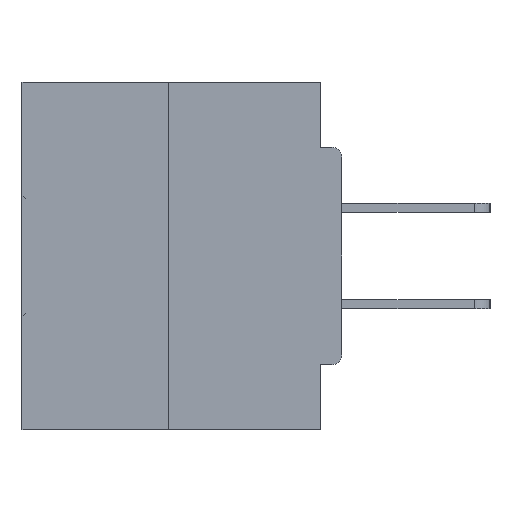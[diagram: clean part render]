
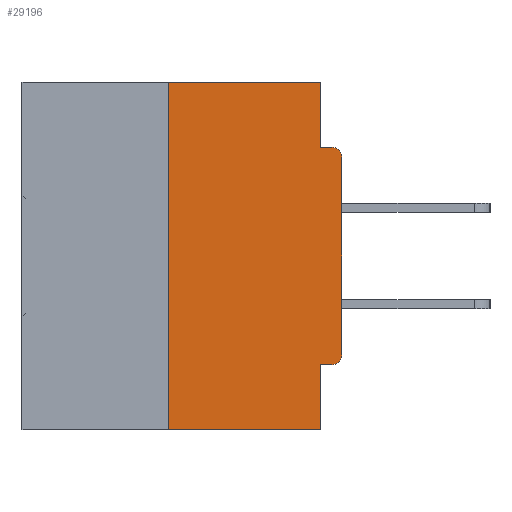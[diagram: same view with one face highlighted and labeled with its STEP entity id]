
A CAD part, left-side view. The second image highlights one B-rep face of the part: STEP entity #29196.
In plain terms, the highlighted planar face has unit normal (-1, 0, 0).
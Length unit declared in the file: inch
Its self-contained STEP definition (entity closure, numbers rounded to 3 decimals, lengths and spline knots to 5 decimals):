
#55 = FACE_OUTER_BOUND ( 'NONE', #29876, .T. ) ;
#307 = VERTEX_POINT ( 'NONE', #12063 ) ;
#422 = VECTOR ( 'NONE', #13585, 39.37008 ) ;
#496 = DIRECTION ( 'NONE',  ( 0., 0., -1. ) ) ;
#652 = CARTESIAN_POINT ( 'NONE',  ( 0., 0.031, 0. ) ) ;
#930 = LINE ( 'NONE', #10908, #422 ) ;
#2035 = DIRECTION ( 'NONE',  ( -1., 0., 0. ) ) ;
#3296 = ORIENTED_EDGE ( 'NONE', *, *, #38791, .F. ) ;
#4219 = EDGE_CURVE ( 'NONE', #8101, #42566, #31066, .T. ) ;
#5062 = ORIENTED_EDGE ( 'NONE', *, *, #29926, .T. ) ;
#5586 = DIRECTION ( 'NONE',  ( 0., 0., -1. ) ) ;
#6471 = DIRECTION ( 'NONE',  ( 1., 0., 0. ) ) ;
#7064 = LINE ( 'NONE', #11049, #9566 ) ;
#7472 = VECTOR ( 'NONE', #21072, 39.37008 ) ;
#7932 = ORIENTED_EDGE ( 'NONE', *, *, #4219, .F. ) ;
#7961 = VERTEX_POINT ( 'NONE', #36113 ) ;
#7991 = DIRECTION ( 'NONE',  ( 0., 1., 0. ) ) ;
#8101 = VERTEX_POINT ( 'NONE', #23896 ) ;
#8283 = CARTESIAN_POINT ( 'NONE',  ( 0., 0.015, -0.0935 ) ) ;
#8564 = VERTEX_POINT ( 'NONE', #42019 ) ;
#8999 = CARTESIAN_POINT ( 'NONE',  ( 0., 0., 0. ) ) ;
#9387 = CIRCLE ( 'NONE', #21454, 0.015 ) ;
#9566 = VECTOR ( 'NONE', #41046, 39.37008 ) ;
#9728 = CARTESIAN_POINT ( 'NONE',  ( 0., 0.031, -0.5 ) ) ;
#9814 = DIRECTION ( 'NONE',  ( -1., 0., 0. ) ) ;
#9816 = VERTEX_POINT ( 'NONE', #8283 ) ;
#10243 = LINE ( 'NONE', #39801, #36415 ) ;
#10625 = VERTEX_POINT ( 'NONE', #31506 ) ;
#10864 = VECTOR ( 'NONE', #35394, 39.37008 ) ;
#10908 = CARTESIAN_POINT ( 'NONE',  ( 0., 0., -0.0935 ) ) ;
#11049 = CARTESIAN_POINT ( 'NONE',  ( 0., 0.25, 0. ) ) ;
#12063 = CARTESIAN_POINT ( 'NONE',  ( 0., 0., -0.3915 ) ) ;
#12364 = ORIENTED_EDGE ( 'NONE', *, *, #25014, .F. ) ;
#13346 = CARTESIAN_POINT ( 'NONE',  ( 0., 0.031, -0.5 ) ) ;
#13406 = EDGE_CURVE ( 'NONE', #42566, #9816, #930, .T. ) ;
#13421 = LINE ( 'NONE', #20533, #18988 ) ;
#13585 = DIRECTION ( 'NONE',  ( 0., -1., 0. ) ) ;
#13755 = ORIENTED_EDGE ( 'NONE', *, *, #36612, .F. ) ;
#16016 = ORIENTED_EDGE ( 'NONE', *, *, #32599, .F. ) ;
#16123 = DIRECTION ( 'NONE',  ( 0., 0., 1. ) ) ;
#16405 = LINE ( 'NONE', #9728, #33679 ) ;
#16942 = PLANE ( 'NONE',  #22169 ) ;
#17149 = DIRECTION ( 'NONE',  ( 0., 0., -1. ) ) ;
#18069 = CARTESIAN_POINT ( 'NONE',  ( 0., 0.25, -0.5 ) ) ;
#18296 = AXIS2_PLACEMENT_3D ( 'NONE', #42648, #2035, #5586 ) ;
#18988 = VECTOR ( 'NONE', #7991, 39.37008 ) ;
#19412 = LINE ( 'NONE', #21879, #10864 ) ;
#20533 = CARTESIAN_POINT ( 'NONE',  ( 0., 0., -0.4065 ) ) ;
#20897 = VERTEX_POINT ( 'NONE', #13346 ) ;
#21072 = DIRECTION ( 'NONE',  ( 0., 0., -1. ) ) ;
#21454 = AXIS2_PLACEMENT_3D ( 'NONE', #26690, #9814, #17149 ) ;
#21879 = CARTESIAN_POINT ( 'NONE',  ( 0., 0.46, -0.5 ) ) ;
#22169 = AXIS2_PLACEMENT_3D ( 'NONE', #30465, #6471, #496 ) ;
#22539 = VERTEX_POINT ( 'NONE', #18069 ) ;
#23295 = DIRECTION ( 'NONE',  ( 0., 0., -1. ) ) ;
#23896 = CARTESIAN_POINT ( 'NONE',  ( 0., 0.031, 0. ) ) ;
#24328 = CARTESIAN_POINT ( 'NONE',  ( 0., 0.031, -0.4065 ) ) ;
#25014 = EDGE_CURVE ( 'NONE', #8564, #8101, #10243, .T. ) ;
#26690 = CARTESIAN_POINT ( 'NONE',  ( 0., 0.015, -0.1085 ) ) ;
#29196 = ADVANCED_FACE ( 'NONE', ( #55 ), #16942, .F. ) ;
#29207 = EDGE_CURVE ( 'NONE', #10625, #9816, #9387, .T. ) ;
#29876 = EDGE_LOOP ( 'NONE', ( #12364, #16016, #41097, #13755, #3296, #37667, #5062, #43112, #40499, #7932 ) ) ;
#29926 = EDGE_CURVE ( 'NONE', #307, #10625, #39427, .T. ) ;
#30025 = DIRECTION ( 'NONE',  ( 0., -1., 0. ) ) ;
#30465 = CARTESIAN_POINT ( 'NONE',  ( 0., 0.46, 0. ) ) ;
#31066 = LINE ( 'NONE', #652, #7472 ) ;
#31506 = CARTESIAN_POINT ( 'NONE',  ( 0., 0., -0.1085 ) ) ;
#32599 = EDGE_CURVE ( 'NONE', #22539, #8564, #7064, .T. ) ;
#32682 = VERTEX_POINT ( 'NONE', #24328 ) ;
#33679 = VECTOR ( 'NONE', #23295, 39.37008 ) ;
#33873 = CIRCLE ( 'NONE', #18296, 0.015 ) ;
#35394 = DIRECTION ( 'NONE',  ( 0., -1., 0. ) ) ;
#35541 = EDGE_CURVE ( 'NONE', #22539, #20897, #19412, .T. ) ;
#36113 = CARTESIAN_POINT ( 'NONE',  ( 0., 0.015, -0.4065 ) ) ;
#36415 = VECTOR ( 'NONE', #30025, 39.37008 ) ;
#36612 = EDGE_CURVE ( 'NONE', #32682, #20897, #16405, .T. ) ;
#37115 = VECTOR ( 'NONE', #16123, 39.37008 ) ;
#37667 = ORIENTED_EDGE ( 'NONE', *, *, #39651, .T. ) ;
#38791 = EDGE_CURVE ( 'NONE', #7961, #32682, #13421, .T. ) ;
#39427 = LINE ( 'NONE', #8999, #37115 ) ;
#39510 = CARTESIAN_POINT ( 'NONE',  ( 0., 0.031, -0.0935 ) ) ;
#39651 = EDGE_CURVE ( 'NONE', #7961, #307, #33873, .T. ) ;
#39801 = CARTESIAN_POINT ( 'NONE',  ( 0., 0.46, 0. ) ) ;
#40499 = ORIENTED_EDGE ( 'NONE', *, *, #13406, .F. ) ;
#41046 = DIRECTION ( 'NONE',  ( 0., 0., 1. ) ) ;
#41097 = ORIENTED_EDGE ( 'NONE', *, *, #35541, .T. ) ;
#42019 = CARTESIAN_POINT ( 'NONE',  ( 0., 0.25, 0. ) ) ;
#42566 = VERTEX_POINT ( 'NONE', #39510 ) ;
#42648 = CARTESIAN_POINT ( 'NONE',  ( 0., 0.015, -0.3915 ) ) ;
#43112 = ORIENTED_EDGE ( 'NONE', *, *, #29207, .T. ) ;
